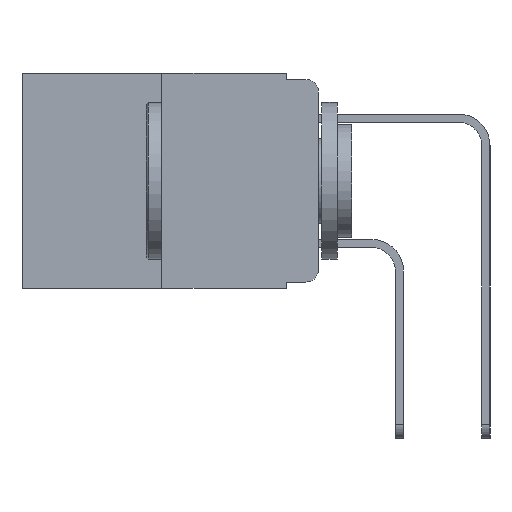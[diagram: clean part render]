
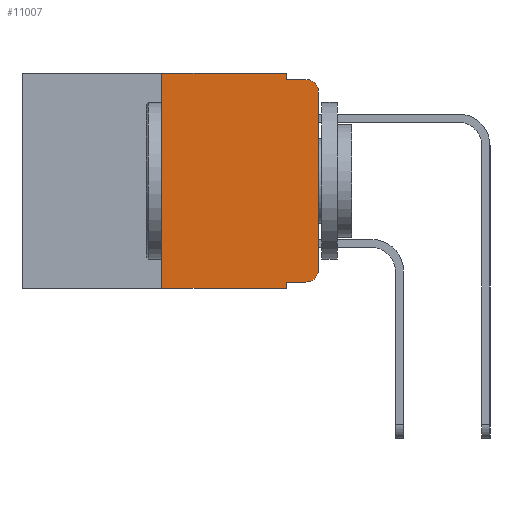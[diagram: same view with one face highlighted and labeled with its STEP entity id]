
A CAD part, left-side view. The second image highlights one B-rep face of the part: STEP entity #11007.
In plain terms, the highlighted planar face has unit normal (-1, 0, 0).
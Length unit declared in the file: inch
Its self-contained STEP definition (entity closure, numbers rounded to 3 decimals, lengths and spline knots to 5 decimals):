
#361 = AXIS2_PLACEMENT_3D ( 'NONE', #8699, #991, #9992 ) ;
#413 = DIRECTION ( 'NONE',  ( 1., 0., 0. ) ) ;
#516 = DIRECTION ( 'NONE',  ( 0., 0., 1. ) ) ;
#535 = EDGE_CURVE ( 'NONE', #8270, #2884, #12719, .T. ) ;
#707 = EDGE_CURVE ( 'NONE', #4698, #1634, #7422, .T. ) ;
#894 = LINE ( 'NONE', #14161, #14123 ) ;
#977 = ORIENTED_EDGE ( 'NONE', *, *, #6939, .F. ) ;
#991 = DIRECTION ( 'NONE',  ( -1., 0., 0. ) ) ;
#1008 = CARTESIAN_POINT ( 'NONE',  ( 0., 0.051, 0. ) ) ;
#1035 = LINE ( 'NONE', #1008, #7902 ) ;
#1075 = CARTESIAN_POINT ( 'NONE',  ( 0., 0.051, -0.333 ) ) ;
#1512 = CARTESIAN_POINT ( 'NONE',  ( 0., 0.02, -0.01 ) ) ;
#1634 = VERTEX_POINT ( 'NONE', #9405 ) ;
#1861 = LINE ( 'NONE', #7863, #11684 ) ;
#2218 = VECTOR ( 'NONE', #516, 39.37008 ) ;
#2297 = VERTEX_POINT ( 'NONE', #9763 ) ;
#2317 = DIRECTION ( 'NONE',  ( 0., 0., -1. ) ) ;
#2410 = VERTEX_POINT ( 'NONE', #4057 ) ;
#2499 = VECTOR ( 'NONE', #15175, 39.37008 ) ;
#2633 = VECTOR ( 'NONE', #7557, 39.37008 ) ;
#2884 = VERTEX_POINT ( 'NONE', #13252 ) ;
#2912 = CARTESIAN_POINT ( 'NONE',  ( 0., 0.02, -0.03 ) ) ;
#3206 = ORIENTED_EDGE ( 'NONE', *, *, #15046, .F. ) ;
#3605 = ORIENTED_EDGE ( 'NONE', *, *, #12363, .F. ) ;
#3633 = CARTESIAN_POINT ( 'NONE',  ( 0., 0.25, -0.343 ) ) ;
#4057 = CARTESIAN_POINT ( 'NONE',  ( 0., 0., -0.313 ) ) ;
#4198 = FACE_OUTER_BOUND ( 'NONE', #13750, .T. ) ;
#4230 = DIRECTION ( 'NONE',  ( 0., 0., -1. ) ) ;
#4698 = VERTEX_POINT ( 'NONE', #10005 ) ;
#4859 = ORIENTED_EDGE ( 'NONE', *, *, #7560, .T. ) ;
#5018 = CIRCLE ( 'NONE', #6323, 0.02 ) ;
#5427 = EDGE_CURVE ( 'NONE', #8223, #12189, #1861, .T. ) ;
#5431 = CARTESIAN_POINT ( 'NONE',  ( 0., 0., -0.03 ) ) ;
#5680 = LINE ( 'NONE', #14596, #2218 ) ;
#5862 = DIRECTION ( 'NONE',  ( 0., -1., 0. ) ) ;
#6068 = CARTESIAN_POINT ( 'NONE',  ( 0., 0.051, -0.01 ) ) ;
#6229 = ORIENTED_EDGE ( 'NONE', *, *, #6670, .T. ) ;
#6279 = CARTESIAN_POINT ( 'NONE',  ( 0., 0.051, 0. ) ) ;
#6323 = AXIS2_PLACEMENT_3D ( 'NONE', #2912, #11866, #4230 ) ;
#6511 = DIRECTION ( 'NONE',  ( 0., 0., 1. ) ) ;
#6670 = EDGE_CURVE ( 'NONE', #2410, #13996, #5680, .T. ) ;
#6939 = EDGE_CURVE ( 'NONE', #4698, #2884, #1035, .T. ) ;
#7422 = LINE ( 'NONE', #1075, #10041 ) ;
#7557 = DIRECTION ( 'NONE',  ( 0., 0., -1. ) ) ;
#7560 = EDGE_CURVE ( 'NONE', #1634, #2410, #12659, .T. ) ;
#7833 = ORIENTED_EDGE ( 'NONE', *, *, #707, .T. ) ;
#7863 = CARTESIAN_POINT ( 'NONE',  ( 0., 0.051, -0.01 ) ) ;
#7902 = VECTOR ( 'NONE', #2317, 39.37008 ) ;
#8140 = CARTESIAN_POINT ( 'NONE',  ( 0., 0.473, 0. ) ) ;
#8223 = VERTEX_POINT ( 'NONE', #6068 ) ;
#8270 = VERTEX_POINT ( 'NONE', #3633 ) ;
#8699 = CARTESIAN_POINT ( 'NONE',  ( 0., 0.02, -0.313 ) ) ;
#9405 = CARTESIAN_POINT ( 'NONE',  ( 0., 0.02, -0.333 ) ) ;
#9407 = DIRECTION ( 'NONE',  ( 0., 0., -1. ) ) ;
#9626 = ORIENTED_EDGE ( 'NONE', *, *, #10956, .T. ) ;
#9701 = CARTESIAN_POINT ( 'NONE',  ( 0., 0.473, 0. ) ) ;
#9763 = CARTESIAN_POINT ( 'NONE',  ( 0., 0.25, 0. ) ) ;
#9992 = DIRECTION ( 'NONE',  ( 0., 0., -1. ) ) ;
#10005 = CARTESIAN_POINT ( 'NONE',  ( 0., 0.051, -0.333 ) ) ;
#10041 = VECTOR ( 'NONE', #14226, 39.37008 ) ;
#10664 = LINE ( 'NONE', #6279, #2633 ) ;
#10832 = ORIENTED_EDGE ( 'NONE', *, *, #535, .T. ) ;
#10956 = EDGE_CURVE ( 'NONE', #13996, #12189, #5018, .T. ) ;
#11007 = ADVANCED_FACE ( 'NONE', ( #4198 ), #11920, .F. ) ;
#11684 = VECTOR ( 'NONE', #14155, 39.37008 ) ;
#11701 = CARTESIAN_POINT ( 'NONE',  ( 0., 0.051, 0. ) ) ;
#11866 = DIRECTION ( 'NONE',  ( -1., 0., 0. ) ) ;
#11920 = PLANE ( 'NONE',  #12323 ) ;
#12094 = EDGE_CURVE ( 'NONE', #8270, #2297, #894, .T. ) ;
#12189 = VERTEX_POINT ( 'NONE', #1512 ) ;
#12323 = AXIS2_PLACEMENT_3D ( 'NONE', #8140, #413, #9407 ) ;
#12363 = EDGE_CURVE ( 'NONE', #2297, #13982, #13115, .T. ) ;
#12659 = CIRCLE ( 'NONE', #361, 0.02 ) ;
#12719 = LINE ( 'NONE', #15812, #2499 ) ;
#13008 = ORIENTED_EDGE ( 'NONE', *, *, #5427, .F. ) ;
#13115 = LINE ( 'NONE', #9701, #16093 ) ;
#13252 = CARTESIAN_POINT ( 'NONE',  ( 0., 0.051, -0.343 ) ) ;
#13750 = EDGE_LOOP ( 'NONE', ( #6229, #9626, #13008, #3206, #3605, #13817, #10832, #977, #7833, #4859 ) ) ;
#13817 = ORIENTED_EDGE ( 'NONE', *, *, #12094, .F. ) ;
#13982 = VERTEX_POINT ( 'NONE', #11701 ) ;
#13996 = VERTEX_POINT ( 'NONE', #5431 ) ;
#14123 = VECTOR ( 'NONE', #6511, 39.37008 ) ;
#14155 = DIRECTION ( 'NONE',  ( 0., -1., 0. ) ) ;
#14161 = CARTESIAN_POINT ( 'NONE',  ( 0., 0.25, 0. ) ) ;
#14226 = DIRECTION ( 'NONE',  ( 0., -1., 0. ) ) ;
#14596 = CARTESIAN_POINT ( 'NONE',  ( 0., 0., 0. ) ) ;
#15046 = EDGE_CURVE ( 'NONE', #13982, #8223, #10664, .T. ) ;
#15175 = DIRECTION ( 'NONE',  ( 0., -1., 0. ) ) ;
#15812 = CARTESIAN_POINT ( 'NONE',  ( 0., 0.473, -0.343 ) ) ;
#16093 = VECTOR ( 'NONE', #5862, 39.37008 ) ;
